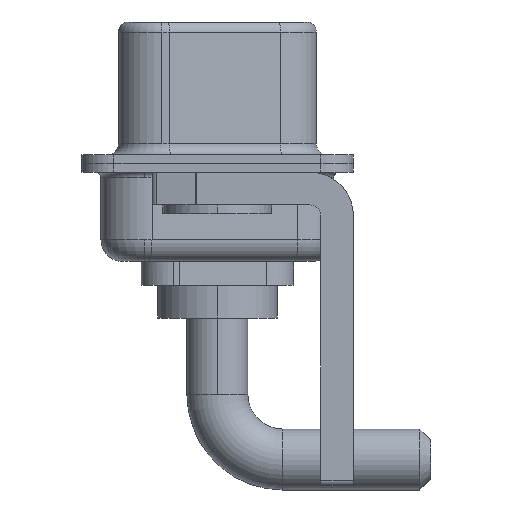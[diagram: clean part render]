
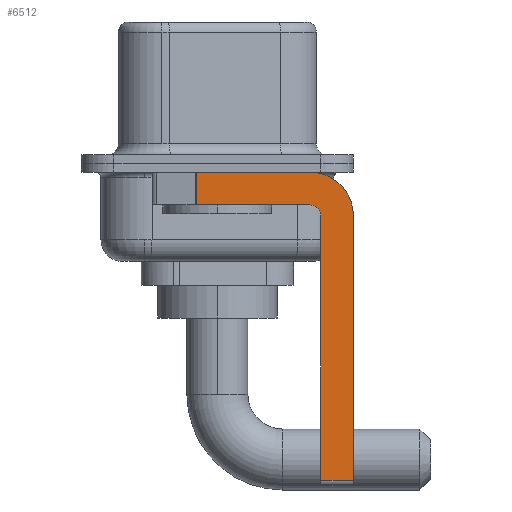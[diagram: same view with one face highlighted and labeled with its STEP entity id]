
A CAD part, left-side view. The second image highlights one B-rep face of the part: STEP entity #6512.
In plain terms, the highlighted planar face has unit normal (-1, 0, 0).
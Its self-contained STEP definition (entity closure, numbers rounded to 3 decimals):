
#6 = CARTESIAN_POINT ( 'NONE',  ( -2.9, 0.978, -0.4 ) ) ;
#14 = DIRECTION ( 'NONE',  ( 0., 0., -1. ) ) ;
#694 = VERTEX_POINT ( 'NONE', #15575 ) ;
#1197 = AXIS2_PLACEMENT_3D ( 'NONE', #9546, #6043, #11123 ) ;
#1208 = CARTESIAN_POINT ( 'NONE',  ( -2.9, -4.25, -0.4 ) ) ;
#1411 = VECTOR ( 'NONE', #16140, 1000. ) ;
#1547 = CARTESIAN_POINT ( 'NONE',  ( -2.9, -6.25, -14.55 ) ) ;
#1566 = AXIS2_PLACEMENT_3D ( 'NONE', #14067, #4991, #14 ) ;
#1727 = EDGE_CURVE ( 'NONE', #4206, #694, #13457, .T. ) ;
#2141 = EDGE_CURVE ( 'NONE', #7568, #6029, #14727, .T. ) ;
#2189 = CARTESIAN_POINT ( 'NONE',  ( -2.9, 0.978, -1.9 ) ) ;
#2530 = EDGE_CURVE ( 'NONE', #6029, #2816, #13137, .T. ) ;
#2612 = DIRECTION ( 'NONE',  ( 0., 0., -1. ) ) ;
#2816 = VERTEX_POINT ( 'NONE', #13037 ) ;
#2837 = ORIENTED_EDGE ( 'NONE', *, *, #8079, .F. ) ;
#2977 = ORIENTED_EDGE ( 'NONE', *, *, #12360, .F. ) ;
#3334 = CARTESIAN_POINT ( 'NONE',  ( -2.9, -4.25, -14.55 ) ) ;
#3369 = DIRECTION ( 'NONE',  ( 0., 0., 1. ) ) ;
#3417 = LINE ( 'NONE', #3334, #8855 ) ;
#4072 = EDGE_CURVE ( 'NONE', #694, #10874, #14046, .T. ) ;
#4206 = VERTEX_POINT ( 'NONE', #8040 ) ;
#4462 = EDGE_LOOP ( 'NONE', ( #10295, #5101, #10938, #7704, #2837, #9947, #2977, #5757 ) ) ;
#4736 = DIRECTION ( 'NONE',  ( 0., -1., 0. ) ) ;
#4991 = DIRECTION ( 'NONE',  ( 1., 0., 0. ) ) ;
#5101 = ORIENTED_EDGE ( 'NONE', *, *, #12659, .T. ) ;
#5244 = CARTESIAN_POINT ( 'NONE',  ( -2.9, -6.25, -2.4 ) ) ;
#5295 = LINE ( 'NONE', #10375, #14557 ) ;
#5757 = ORIENTED_EDGE ( 'NONE', *, *, #2530, .F. ) ;
#5977 = CARTESIAN_POINT ( 'NONE',  ( -2.9, 3., -0.4 ) ) ;
#6029 = VERTEX_POINT ( 'NONE', #1208 ) ;
#6043 = DIRECTION ( 'NONE',  ( 1., 0., 0. ) ) ;
#6512 = ADVANCED_FACE ( 'NONE', ( #8815 ), #16409, .F. ) ;
#6770 = VECTOR ( 'NONE', #14125, 1000. ) ;
#7233 = AXIS2_PLACEMENT_3D ( 'NONE', #13659, #14914, #3369 ) ;
#7384 = VECTOR ( 'NONE', #11054, 1000. ) ;
#7568 = VERTEX_POINT ( 'NONE', #6 ) ;
#7704 = ORIENTED_EDGE ( 'NONE', *, *, #1727, .F. ) ;
#8040 = CARTESIAN_POINT ( 'NONE',  ( -2.9, -4.75, -2.4 ) ) ;
#8079 = EDGE_CURVE ( 'NONE', #12620, #4206, #5295, .T. ) ;
#8282 = VECTOR ( 'NONE', #2612, 1000. ) ;
#8561 = LINE ( 'NONE', #15055, #1411 ) ;
#8815 = FACE_OUTER_BOUND ( 'NONE', #4462, .T. ) ;
#8855 = VECTOR ( 'NONE', #4736, 1000. ) ;
#9546 = CARTESIAN_POINT ( 'NONE',  ( -2.9, -4.25, -2.4 ) ) ;
#9947 = ORIENTED_EDGE ( 'NONE', *, *, #15053, .T. ) ;
#10295 = ORIENTED_EDGE ( 'NONE', *, *, #2141, .F. ) ;
#10375 = CARTESIAN_POINT ( 'NONE',  ( -2.9, -4.75, -14.8 ) ) ;
#10874 = VERTEX_POINT ( 'NONE', #2189 ) ;
#10938 = ORIENTED_EDGE ( 'NONE', *, *, #4072, .F. ) ;
#11054 = DIRECTION ( 'NONE',  ( 0., -1., 0. ) ) ;
#11123 = DIRECTION ( 'NONE',  ( 0., 0., -1. ) ) ;
#11449 = CARTESIAN_POINT ( 'NONE',  ( -2.9, -4.25, -1.9 ) ) ;
#11729 = LINE ( 'NONE', #5244, #8282 ) ;
#11852 = VERTEX_POINT ( 'NONE', #1547 ) ;
#12360 = EDGE_CURVE ( 'NONE', #2816, #11852, #11729, .T. ) ;
#12463 = CARTESIAN_POINT ( 'NONE',  ( -2.9, -4.75, -14.55 ) ) ;
#12620 = VERTEX_POINT ( 'NONE', #12463 ) ;
#12659 = EDGE_CURVE ( 'NONE', #7568, #10874, #8561, .T. ) ;
#13037 = CARTESIAN_POINT ( 'NONE',  ( -2.9, -6.25, -2.4 ) ) ;
#13137 = CIRCLE ( 'NONE', #1197, 2. ) ;
#13457 = CIRCLE ( 'NONE', #7233, 0.5 ) ;
#13659 = CARTESIAN_POINT ( 'NONE',  ( -2.9, -4.25, -2.4 ) ) ;
#13873 = DIRECTION ( 'NONE',  ( 0., 0., 1. ) ) ;
#14046 = LINE ( 'NONE', #11449, #6770 ) ;
#14067 = CARTESIAN_POINT ( 'NONE',  ( -2.9, -4.25, -2.4 ) ) ;
#14125 = DIRECTION ( 'NONE',  ( 0., 1., 0. ) ) ;
#14557 = VECTOR ( 'NONE', #13873, 1000. ) ;
#14727 = LINE ( 'NONE', #5977, #7384 ) ;
#14914 = DIRECTION ( 'NONE',  ( -1., 0., 0. ) ) ;
#15053 = EDGE_CURVE ( 'NONE', #12620, #11852, #3417, .T. ) ;
#15055 = CARTESIAN_POINT ( 'NONE',  ( -2.9, 0.978, -1.9 ) ) ;
#15575 = CARTESIAN_POINT ( 'NONE',  ( -2.9, -4.25, -1.9 ) ) ;
#16140 = DIRECTION ( 'NONE',  ( 0., 0., -1. ) ) ;
#16409 = PLANE ( 'NONE',  #1566 ) ;
